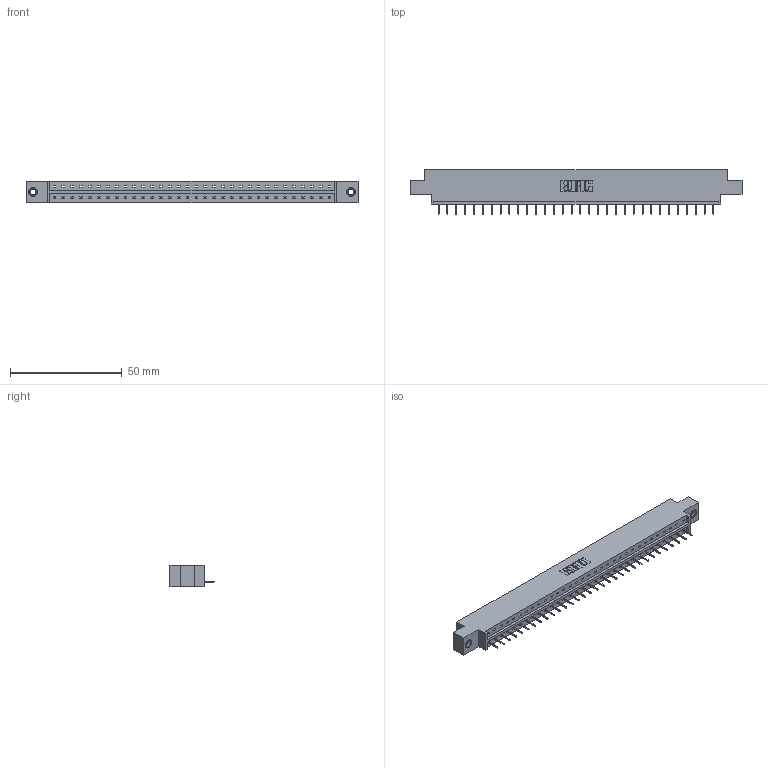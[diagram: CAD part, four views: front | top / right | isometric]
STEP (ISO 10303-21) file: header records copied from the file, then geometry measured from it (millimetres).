
FILE_DESCRIPTION (( 'STEP AP203' ), '1' );
FILE_NAME ('333-032-524-607.STEP', '2018-08-02T20:04:13', ( '' ), ( '' ), 'SwSTEP 2.0', 'SolidWorks 2016', '' );
FILE_SCHEMA (( 'CONFIG_CONTROL_DESIGN' ));
Length unit declared in the file: inch
Products named in the file (4): 333 Part_Offset - .156 Dia - TI; 345-292-001_345-293-124; 345-250-001_345-250-005-103; 333-032-524-607
Assembly tree (35 placements, depth 2):
  333-032-524-607
    333 Part_Offset - .156 Dia - TI
    345-292-001_345-293-124  x32
    345-250-001_345-250-005-103  x2
Bounding box: 148.34 x 19.69 x 9.4 mm (x, y, z)
Volume: 14473.1 mm3; surface area: 15395.3 mm2
Topology: 35 solids, 35 shells, 2162 faces, 6219 edges, 4010 vertices
Faces by surface type: plane 1642, cylinder 504, cone 12, torus 4
Entity records: 22248 total; most frequent: CARTESIAN_POINT 3821, ORIENTED_EDGE 3782, DIRECTION 3277, EDGE_CURVE 1891, LINE 1747, VECTOR 1747, VERTEX_POINT 1252, AXIS2_PLACEMENT_3D 765
